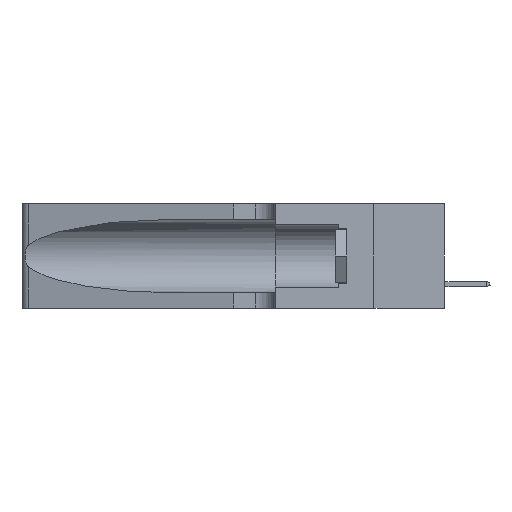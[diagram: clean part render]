
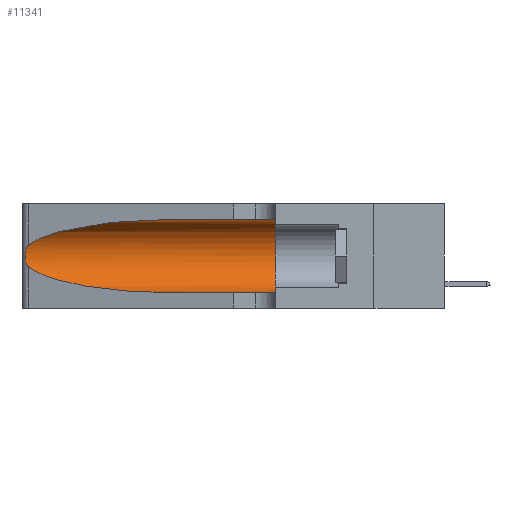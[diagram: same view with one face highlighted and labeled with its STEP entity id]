
A CAD part, left-side view. The second image highlights one B-rep face of the part: STEP entity #11341.
In plain terms, the highlighted cylindrical face has radius 3.308 mm (diameter 6.617 mm), a partial arc.
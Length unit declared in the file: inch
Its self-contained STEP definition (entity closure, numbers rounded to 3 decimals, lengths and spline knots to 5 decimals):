
#14 = VERTEX_POINT ( 'NONE', #5424 ) ;
#331 = CARTESIAN_POINT ( 'NONE',  ( 0.25639, 1.23186, 0.15144 ) ) ;
#518 = FACE_OUTER_BOUND ( 'NONE', #14666, .T. ) ;
#1269 = CARTESIAN_POINT ( 'NONE',  ( 0.2373, 1.15595, 0.08982 ) ) ;
#2501 = CYLINDRICAL_SURFACE ( 'NONE', #18096, 0.13025 ) ;
#2652 = CARTESIAN_POINT ( 'NONE',  ( 0.1305, 0.35, 0.31525 ) ) ;
#2781 =( BOUNDED_CURVE ( )  B_SPLINE_CURVE ( 3, ( #20433, #1269, #5549, #20702 ),
 .UNSPECIFIED., .F., .T. ) 
 B_SPLINE_CURVE_WITH_KNOTS ( ( 4, 4 ),
 ( 3.44316, 4.71239 ),
 .UNSPECIFIED. ) 
 CURVE ( )  GEOMETRIC_REPRESENTATION_ITEM ( )  RATIONAL_B_SPLINE_CURVE ( ( 1., 0.87, 0.87, 1. ) ) 
 REPRESENTATION_ITEM ( '' )  );
#3803 = CARTESIAN_POINT ( 'NONE',  ( 0.1305, 0.35, 0.05475 ) ) ;
#5060 = CARTESIAN_POINT ( 'NONE',  ( 0.25487, 1.22718, 0.14631 ) ) ;
#5424 = CARTESIAN_POINT ( 'NONE',  ( 0.1305, 0.72297, 0.05475 ) ) ;
#5549 = CARTESIAN_POINT ( 'NONE',  ( 0.18966, 0.96281, 0.05475 ) ) ;
#5802 = VECTOR ( 'NONE', #7349, 39.37008 ) ;
#6578 = CARTESIAN_POINT ( 'NONE',  ( 0.25555, 1.22994, 0.2215 ) ) ;
#7334 = CARTESIAN_POINT ( 'NONE',  ( 0.2373, 1.15595, 0.28018 ) ) ;
#7349 = DIRECTION ( 'NONE',  ( 0., -1., 0. ) ) ;
#7900 = VERTEX_POINT ( 'NONE', #5060 ) ;
#8002 = ORIENTED_EDGE ( 'NONE', *, *, #8219, .T. ) ;
#8063 = DIRECTION ( 'NONE',  ( 0., 0., -1. ) ) ;
#8219 = EDGE_CURVE ( 'NONE', #26484, #25150, #26760, .T. ) ;
#8601 = B_SPLINE_CURVE_WITH_KNOTS ( 'NONE', 3,
 ( #8718, #6578, #23660, #10848, #19587, #17240, #21713, #25635, #17140, #25903, #14977, #331, #23563, #25819 ),
 .UNSPECIFIED., .F., .F.,
 ( 4, 2, 2, 2, 2, 2, 4 ),
 ( 0., 0.00027, 0.00053, 0.00107, 0.0016, 0.00187, 0.00214 ),
 .UNSPECIFIED. ) ;
#8605 = CARTESIAN_POINT ( 'NONE',  ( 0.1305, 0.35, 0.185 ) ) ;
#8718 = CARTESIAN_POINT ( 'NONE',  ( 0.25487, 1.22718, 0.22369 ) ) ;
#9383 = CARTESIAN_POINT ( 'NONE',  ( 0.1305, 0.72297, 0.31525 ) ) ;
#9523 = VECTOR ( 'NONE', #27321, 39.37008 ) ;
#10444 = LINE ( 'NONE', #18023, #5802 ) ;
#10848 = CARTESIAN_POINT ( 'NONE',  ( 0.25787, 1.23484, 0.2124 ) ) ;
#11110 = VERTEX_POINT ( 'NONE', #2652 ) ;
#11242 = EDGE_CURVE ( 'NONE', #7900, #14, #2781, .T. ) ;
#11341 = ADVANCED_FACE ( 'NONE', ( #518 ), #2501, .F. ) ;
#13236 = EDGE_CURVE ( 'NONE', #11110, #26098, #19014, .T. ) ;
#13264 = DIRECTION ( 'NONE',  ( 0., 0., 1. ) ) ;
#13692 = CARTESIAN_POINT ( 'NONE',  ( 0.18966, 0.96281, 0.31525 ) ) ;
#14152 = ORIENTED_EDGE ( 'NONE', *, *, #15135, .T. ) ;
#14666 = EDGE_LOOP ( 'NONE', ( #8002, #14152, #21464, #21360, #18744, #17697 ) ) ;
#14977 = CARTESIAN_POINT ( 'NONE',  ( 0.25789, 1.23486, 0.15765 ) ) ;
#15135 = EDGE_CURVE ( 'NONE', #25150, #7900, #8601, .T. ) ;
#15244 = DIRECTION ( 'NONE',  ( 0., 1., 0. ) ) ;
#16322 = AXIS2_PLACEMENT_3D ( 'NONE', #8605, #15244, #13264 ) ;
#16667 = CARTESIAN_POINT ( 'NONE',  ( 0.1305, 1.61858, 0.185 ) ) ;
#16760 = DIRECTION ( 'NONE',  ( 0., -1., 0. ) ) ;
#17140 = CARTESIAN_POINT ( 'NONE',  ( 0.26017, 1.23833, 0.17102 ) ) ;
#17240 = CARTESIAN_POINT ( 'NONE',  ( 0.26018, 1.23835, 0.19895 ) ) ;
#17697 = ORIENTED_EDGE ( 'NONE', *, *, #24008, .F. ) ;
#17913 = CARTESIAN_POINT ( 'NONE',  ( 0.1305, 0.72297, 0.31525 ) ) ;
#18023 = CARTESIAN_POINT ( 'NONE',  ( 0.1305, 1.61858, 0.31525 ) ) ;
#18096 = AXIS2_PLACEMENT_3D ( 'NONE', #16667, #16760, #8063 ) ;
#18239 = CARTESIAN_POINT ( 'NONE',  ( 0.25487, 1.22718, 0.22369 ) ) ;
#18609 = LINE ( 'NONE', #18714, #9523 ) ;
#18714 = CARTESIAN_POINT ( 'NONE',  ( 0.1305, 1.61858, 0.05475 ) ) ;
#18744 = ORIENTED_EDGE ( 'NONE', *, *, #13236, .F. ) ;
#19014 = CIRCLE ( 'NONE', #16322, 0.13025 ) ;
#19587 = CARTESIAN_POINT ( 'NONE',  ( 0.25854, 1.2359, 0.20912 ) ) ;
#20433 = CARTESIAN_POINT ( 'NONE',  ( 0.25487, 1.22718, 0.14631 ) ) ;
#20702 = CARTESIAN_POINT ( 'NONE',  ( 0.1305, 0.72297, 0.05475 ) ) ;
#21360 = ORIENTED_EDGE ( 'NONE', *, *, #26127, .T. ) ;
#21464 = ORIENTED_EDGE ( 'NONE', *, *, #11242, .T. ) ;
#21713 = CARTESIAN_POINT ( 'NONE',  ( 0.26075, 1.23896, 0.19203 ) ) ;
#23563 = CARTESIAN_POINT ( 'NONE',  ( 0.25555, 1.22993, 0.14849 ) ) ;
#23660 = CARTESIAN_POINT ( 'NONE',  ( 0.25639, 1.23184, 0.21858 ) ) ;
#24008 = EDGE_CURVE ( 'NONE', #26484, #11110, #10444, .T. ) ;
#25150 = VERTEX_POINT ( 'NONE', #18239 ) ;
#25635 = CARTESIAN_POINT ( 'NONE',  ( 0.26075, 1.23896, 0.178 ) ) ;
#25819 = CARTESIAN_POINT ( 'NONE',  ( 0.25487, 1.22718, 0.14631 ) ) ;
#25903 = CARTESIAN_POINT ( 'NONE',  ( 0.25856, 1.23593, 0.16098 ) ) ;
#26098 = VERTEX_POINT ( 'NONE', #3803 ) ;
#26127 = EDGE_CURVE ( 'NONE', #14, #26098, #18609, .T. ) ;
#26484 = VERTEX_POINT ( 'NONE', #9383 ) ;
#26569 = CARTESIAN_POINT ( 'NONE',  ( 0.25487, 1.22718, 0.22369 ) ) ;
#26760 =( BOUNDED_CURVE ( )  B_SPLINE_CURVE ( 3, ( #17913, #13692, #7334, #26569 ),
 .UNSPECIFIED., .F., .F. ) 
 B_SPLINE_CURVE_WITH_KNOTS ( ( 4, 4 ),
 ( 1.5708, 2.84003 ),
 .UNSPECIFIED. ) 
 CURVE ( )  GEOMETRIC_REPRESENTATION_ITEM ( )  RATIONAL_B_SPLINE_CURVE ( ( 1., 0.87, 0.87, 1. ) ) 
 REPRESENTATION_ITEM ( '' )  );
#27321 = DIRECTION ( 'NONE',  ( 0., -1., 0. ) ) ;
